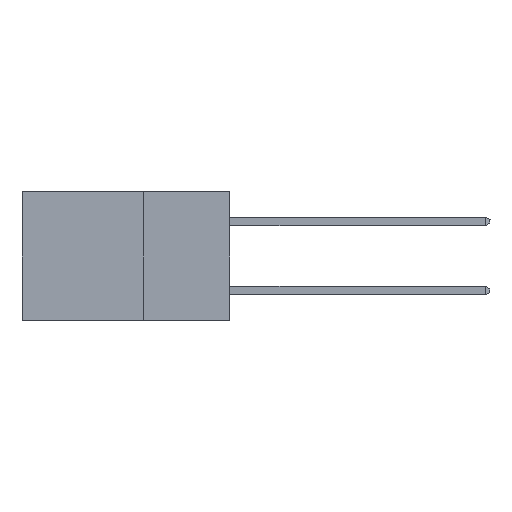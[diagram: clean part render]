
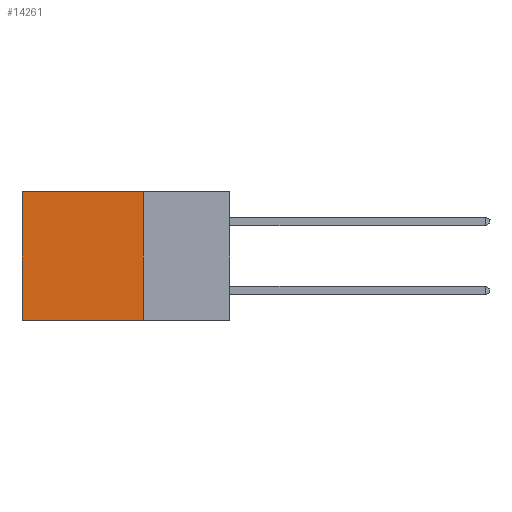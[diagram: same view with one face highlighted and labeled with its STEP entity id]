
A CAD part, left-side view. The second image highlights one B-rep face of the part: STEP entity #14261.
In plain terms, the highlighted planar face has unit normal (-1, 0, 0).
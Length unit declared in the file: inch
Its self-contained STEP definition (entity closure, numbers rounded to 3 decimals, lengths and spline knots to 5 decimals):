
#191 = FACE_OUTER_BOUND ( 'NONE', #7478, .T. ) ;
#1336 = ORIENTED_EDGE ( 'NONE', *, *, #20995, .F. ) ;
#1626 = LINE ( 'NONE', #16220, #5018 ) ;
#2679 = VERTEX_POINT ( 'NONE', #13578 ) ;
#3183 = ORIENTED_EDGE ( 'NONE', *, *, #22815, .T. ) ;
#3925 = LINE ( 'NONE', #9814, #6487 ) ;
#4058 = CARTESIAN_POINT ( 'NONE',  ( 0.2615, 0.25, -0.37 ) ) ;
#4074 = LINE ( 'NONE', #20010, #18630 ) ;
#5018 = VECTOR ( 'NONE', #11934, 39.37008 ) ;
#5720 = DIRECTION ( 'NONE',  ( 1., 0., 0. ) ) ;
#6487 = VECTOR ( 'NONE', #16231, 39.37008 ) ;
#7478 = EDGE_LOOP ( 'NONE', ( #25130, #1336, #17437, #3183 ) ) ;
#8378 = PLANE ( 'NONE',  #12183 ) ;
#9814 = CARTESIAN_POINT ( 'NONE',  ( 0.2615, 0.6, -0.37 ) ) ;
#10942 = EDGE_CURVE ( 'NONE', #2679, #17742, #3925, .T. ) ;
#11085 = VERTEX_POINT ( 'NONE', #4058 ) ;
#11934 = DIRECTION ( 'NONE',  ( 0., 1., 0. ) ) ;
#12183 = AXIS2_PLACEMENT_3D ( 'NONE', #16284, #5720, #24078 ) ;
#13116 = VECTOR ( 'NONE', #16708, 39.37008 ) ;
#13578 = CARTESIAN_POINT ( 'NONE',  ( 0.2615, 0.6, 0. ) ) ;
#14261 = ADVANCED_FACE ( 'NONE', ( #191 ), #8378, .F. ) ;
#15100 = CARTESIAN_POINT ( 'NONE',  ( 0.2615, 0.25, -0.37 ) ) ;
#16114 = DIRECTION ( 'NONE',  ( 0., 1., 0. ) ) ;
#16220 = CARTESIAN_POINT ( 'NONE',  ( 0.2615, 0.25, 0. ) ) ;
#16231 = DIRECTION ( 'NONE',  ( 0., 0., -1. ) ) ;
#16284 = CARTESIAN_POINT ( 'NONE',  ( 0.2615, 0.25, -0.37 ) ) ;
#16390 = CARTESIAN_POINT ( 'NONE',  ( 0.2615, 0.6, -0.37 ) ) ;
#16708 = DIRECTION ( 'NONE',  ( 0., 0., -1. ) ) ;
#17399 = CARTESIAN_POINT ( 'NONE',  ( 0.2615, 0.25, 0. ) ) ;
#17437 = ORIENTED_EDGE ( 'NONE', *, *, #20282, .F. ) ;
#17742 = VERTEX_POINT ( 'NONE', #16390 ) ;
#18630 = VECTOR ( 'NONE', #16114, 39.37008 ) ;
#20010 = CARTESIAN_POINT ( 'NONE',  ( 0.2615, 0.25, -0.37 ) ) ;
#20282 = EDGE_CURVE ( 'NONE', #21722, #11085, #22895, .T. ) ;
#20995 = EDGE_CURVE ( 'NONE', #11085, #17742, #4074, .T. ) ;
#21722 = VERTEX_POINT ( 'NONE', #17399 ) ;
#22815 = EDGE_CURVE ( 'NONE', #21722, #2679, #1626, .T. ) ;
#22895 = LINE ( 'NONE', #15100, #13116 ) ;
#24078 = DIRECTION ( 'NONE',  ( 0., 0., -1. ) ) ;
#25130 = ORIENTED_EDGE ( 'NONE', *, *, #10942, .T. ) ;
